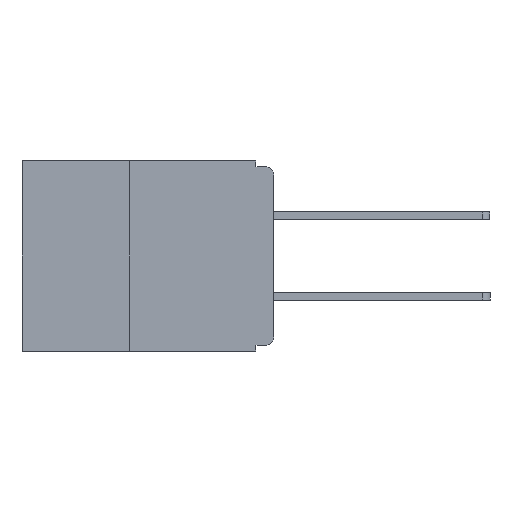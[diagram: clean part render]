
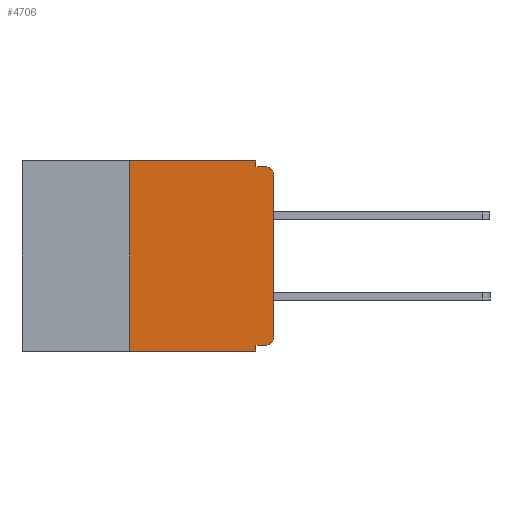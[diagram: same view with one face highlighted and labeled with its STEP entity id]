
A CAD part, left-side view. The second image highlights one B-rep face of the part: STEP entity #4706.
In plain terms, the highlighted planar face has unit normal (-1, 0, 0).
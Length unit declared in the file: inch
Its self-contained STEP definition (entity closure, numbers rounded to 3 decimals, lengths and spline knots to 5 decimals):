
#1478 = EDGE_CURVE ( 'NONE', #24091, #20400, #5166, .T. ) ;
#1694 = VERTEX_POINT ( 'NONE', #13789 ) ;
#1915 = CARTESIAN_POINT ( 'NONE',  ( 0., 0.015, -0.01 ) ) ;
#1984 = DIRECTION ( 'NONE',  ( 0., 0., -1. ) ) ;
#2021 = DIRECTION ( 'NONE',  ( 1., 0., 0. ) ) ;
#2063 = VECTOR ( 'NONE', #24808, 39.37008 ) ;
#2079 = CARTESIAN_POINT ( 'NONE',  ( 0., 0.437, 0. ) ) ;
#2082 = ORIENTED_EDGE ( 'NONE', *, *, #7806, .T. ) ;
#2147 = PLANE ( 'NONE',  #19132 ) ;
#2419 = ORIENTED_EDGE ( 'NONE', *, *, #20713, .T. ) ;
#2486 = FACE_OUTER_BOUND ( 'NONE', #21322, .T. ) ;
#2789 = DIRECTION ( 'NONE',  ( -1., 0., 0. ) ) ;
#2835 = ORIENTED_EDGE ( 'NONE', *, *, #10790, .F. ) ;
#3091 = LINE ( 'NONE', #3859, #23849 ) ;
#3134 = ORIENTED_EDGE ( 'NONE', *, *, #11020, .F. ) ;
#3150 = AXIS2_PLACEMENT_3D ( 'NONE', #14976, #2789, #16962 ) ;
#3407 = CARTESIAN_POINT ( 'NONE',  ( 0., 0., -0.305 ) ) ;
#3539 = ORIENTED_EDGE ( 'NONE', *, *, #19772, .F. ) ;
#3818 = ORIENTED_EDGE ( 'NONE', *, *, #5751, .F. ) ;
#3859 = CARTESIAN_POINT ( 'NONE',  ( 0., 0.437, 0. ) ) ;
#4241 = VECTOR ( 'NONE', #5012, 39.37008 ) ;
#4267 = VECTOR ( 'NONE', #5629, 39.37008 ) ;
#4372 = ORIENTED_EDGE ( 'NONE', *, *, #23196, .T. ) ;
#4506 = ORIENTED_EDGE ( 'NONE', *, *, #1478, .F. ) ;
#4706 = ADVANCED_FACE ( 'NONE', ( #2486 ), #2147, .F. ) ;
#4787 = CARTESIAN_POINT ( 'NONE',  ( 0., 0., -0.01 ) ) ;
#5011 = LINE ( 'NONE', #23555, #15121 ) ;
#5012 = DIRECTION ( 'NONE',  ( 0., 1., 0. ) ) ;
#5166 = LINE ( 'NONE', #6429, #25771 ) ;
#5561 = ORIENTED_EDGE ( 'NONE', *, *, #11452, .F. ) ;
#5629 = DIRECTION ( 'NONE',  ( 0., 0., -1. ) ) ;
#5751 = EDGE_CURVE ( 'NONE', #21326, #9496, #22933, .T. ) ;
#5874 = ORIENTED_EDGE ( 'NONE', *, *, #10345, .T. ) ;
#6429 = CARTESIAN_POINT ( 'NONE',  ( 0., 0.031, -0.33 ) ) ;
#6481 = CARTESIAN_POINT ( 'NONE',  ( 0., 0.015, -0.305 ) ) ;
#6619 = VERTEX_POINT ( 'NONE', #23808 ) ;
#6962 = CARTESIAN_POINT ( 'NONE',  ( 0., 0., -0.32 ) ) ;
#7806 = EDGE_CURVE ( 'NONE', #14855, #19724, #8476, .T. ) ;
#7854 = AXIS2_PLACEMENT_3D ( 'NONE', #6481, #20486, #8597 ) ;
#8476 = LINE ( 'NONE', #18043, #18463 ) ;
#8597 = DIRECTION ( 'NONE',  ( 0., 0., -1. ) ) ;
#9496 = VERTEX_POINT ( 'NONE', #25646 ) ;
#9637 = LINE ( 'NONE', #6962, #4241 ) ;
#9662 = LINE ( 'NONE', #21581, #4267 ) ;
#10345 = EDGE_CURVE ( 'NONE', #6619, #14855, #21763, .T. ) ;
#10790 = EDGE_CURVE ( 'NONE', #1694, #16541, #25255, .T. ) ;
#11020 = EDGE_CURVE ( 'NONE', #17525, #1694, #9662, .T. ) ;
#11452 = EDGE_CURVE ( 'NONE', #6619, #24091, #9637, .T. ) ;
#11754 = CARTESIAN_POINT ( 'NONE',  ( 0., 0.031, 0. ) ) ;
#11948 = CARTESIAN_POINT ( 'NONE',  ( 0., 0.031, -0.32 ) ) ;
#11953 = CIRCLE ( 'NONE', #3150, 0.015 ) ;
#12128 = DIRECTION ( 'NONE',  ( 0., 0., 1. ) ) ;
#13789 = CARTESIAN_POINT ( 'NONE',  ( 0., 0.031, -0.01 ) ) ;
#14721 = VECTOR ( 'NONE', #16844, 39.37008 ) ;
#14855 = VERTEX_POINT ( 'NONE', #3407 ) ;
#14921 = CARTESIAN_POINT ( 'NONE',  ( 0., 0.25, -0.33 ) ) ;
#14976 = CARTESIAN_POINT ( 'NONE',  ( 0., 0.015, -0.025 ) ) ;
#15121 = VECTOR ( 'NONE', #21530, 39.37008 ) ;
#15880 = CARTESIAN_POINT ( 'NONE',  ( 0., 0., -0.025 ) ) ;
#16541 = VERTEX_POINT ( 'NONE', #1915 ) ;
#16844 = DIRECTION ( 'NONE',  ( 0., -1., 0. ) ) ;
#16962 = DIRECTION ( 'NONE',  ( 0., 0., -1. ) ) ;
#17525 = VERTEX_POINT ( 'NONE', #11754 ) ;
#17959 = DIRECTION ( 'NONE',  ( 0., -1., 0. ) ) ;
#18043 = CARTESIAN_POINT ( 'NONE',  ( 0., 0., 0. ) ) ;
#18463 = VECTOR ( 'NONE', #12128, 39.37008 ) ;
#19132 = AXIS2_PLACEMENT_3D ( 'NONE', #2079, #2021, #1984 ) ;
#19724 = VERTEX_POINT ( 'NONE', #15880 ) ;
#19772 = EDGE_CURVE ( 'NONE', #9496, #17525, #3091, .T. ) ;
#19808 = CARTESIAN_POINT ( 'NONE',  ( 0., 0.031, -0.33 ) ) ;
#20400 = VERTEX_POINT ( 'NONE', #19808 ) ;
#20486 = DIRECTION ( 'NONE',  ( -1., 0., 0. ) ) ;
#20713 = EDGE_CURVE ( 'NONE', #19724, #16541, #11953, .T. ) ;
#21322 = EDGE_LOOP ( 'NONE', ( #2082, #2419, #2835, #3134, #3539, #3818, #4372, #4506, #5561, #5874 ) ) ;
#21326 = VERTEX_POINT ( 'NONE', #24756 ) ;
#21530 = DIRECTION ( 'NONE',  ( 0., -1., 0. ) ) ;
#21581 = CARTESIAN_POINT ( 'NONE',  ( 0., 0.031, 0. ) ) ;
#21763 = CIRCLE ( 'NONE', #7854, 0.015 ) ;
#22933 = LINE ( 'NONE', #14921, #2063 ) ;
#23196 = EDGE_CURVE ( 'NONE', #21326, #20400, #5011, .T. ) ;
#23491 = DIRECTION ( 'NONE',  ( 0., 0., -1. ) ) ;
#23555 = CARTESIAN_POINT ( 'NONE',  ( 0., 0.437, -0.33 ) ) ;
#23808 = CARTESIAN_POINT ( 'NONE',  ( 0., 0.015, -0.32 ) ) ;
#23849 = VECTOR ( 'NONE', #17959, 39.37008 ) ;
#24091 = VERTEX_POINT ( 'NONE', #11948 ) ;
#24756 = CARTESIAN_POINT ( 'NONE',  ( 0., 0.25, -0.33 ) ) ;
#24808 = DIRECTION ( 'NONE',  ( 0., 0., 1. ) ) ;
#25255 = LINE ( 'NONE', #4787, #14721 ) ;
#25646 = CARTESIAN_POINT ( 'NONE',  ( 0., 0.25, 0. ) ) ;
#25771 = VECTOR ( 'NONE', #23491, 39.37008 ) ;
